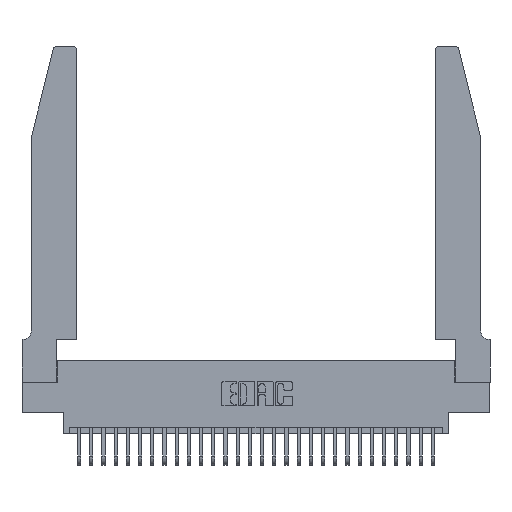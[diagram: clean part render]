
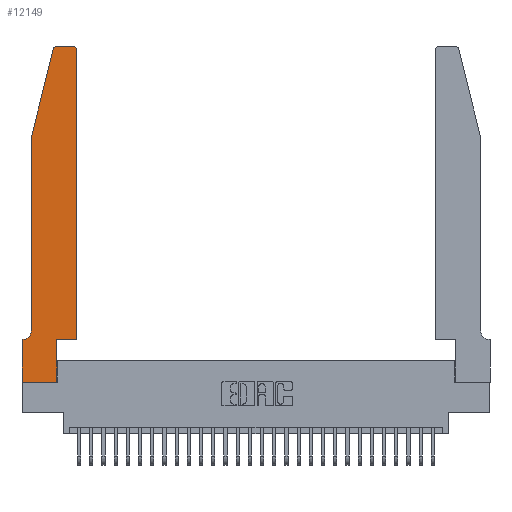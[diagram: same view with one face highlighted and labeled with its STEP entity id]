
A CAD part, top view. The second image highlights one B-rep face of the part: STEP entity #12149.
In plain terms, the highlighted planar face has unit normal (0, 0, 1).
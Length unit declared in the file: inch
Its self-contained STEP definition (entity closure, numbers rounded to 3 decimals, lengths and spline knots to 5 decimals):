
#198 = LINE ( 'NONE', #25534, #5216 ) ;
#710 = DIRECTION ( 'NONE',  ( 0., 0., 1. ) ) ;
#942 = ORIENTED_EDGE ( 'NONE', *, *, #18002, .T. ) ;
#1253 = DIRECTION ( 'NONE',  ( 0., 1., 0. ) ) ;
#2270 = EDGE_CURVE ( 'NONE', #3333, #13601, #4426, .T. ) ;
#2566 = ORIENTED_EDGE ( 'NONE', *, *, #16374, .T. ) ;
#2640 = CARTESIAN_POINT ( 'NONE',  ( 0.0055, 0.42, 0.37 ) ) ;
#3074 = CARTESIAN_POINT ( 'NONE',  ( 0.2865, 0.35, 0.37 ) ) ;
#3125 = DIRECTION ( 'NONE',  ( 0., -1., 0. ) ) ;
#3129 = LINE ( 'NONE', #16320, #8863 ) ;
#3278 = CARTESIAN_POINT ( 'NONE',  ( 0., 0., 0.37 ) ) ;
#3333 = VERTEX_POINT ( 'NONE', #3588 ) ;
#3439 = EDGE_CURVE ( 'NONE', #27283, #3333, #3129, .T. ) ;
#3588 = CARTESIAN_POINT ( 'NONE',  ( 0.0755, 2., 0.37 ) ) ;
#4221 = VECTOR ( 'NONE', #9156, 39.37008 ) ;
#4374 = AXIS2_PLACEMENT_3D ( 'NONE', #2640, #7569, #20020 ) ;
#4426 = LINE ( 'NONE', #17891, #21576 ) ;
#4939 = CARTESIAN_POINT ( 'NONE',  ( 0.4205, 2.75, 0.37 ) ) ;
#4962 = VECTOR ( 'NONE', #5959, 39.37008 ) ;
#5185 = EDGE_CURVE ( 'NONE', #8515, #17104, #23289, .T. ) ;
#5216 = VECTOR ( 'NONE', #20667, 39.37008 ) ;
#5432 = EDGE_CURVE ( 'NONE', #28858, #16392, #21372, .T. ) ;
#5959 = DIRECTION ( 'NONE',  ( -1., 0., 0. ) ) ;
#6767 = CARTESIAN_POINT ( 'NONE',  ( 0., 0.35, 0.37 ) ) ;
#6774 = ORIENTED_EDGE ( 'NONE', *, *, #3439, .T. ) ;
#6834 = CARTESIAN_POINT ( 'NONE',  ( 0.4505, 0.35, 0.37 ) ) ;
#7539 = VECTOR ( 'NONE', #15775, 39.37008 ) ;
#7569 = DIRECTION ( 'NONE',  ( 0., 0., -1. ) ) ;
#7697 = CARTESIAN_POINT ( 'NONE',  ( 0.0755, 0.35, 0.37 ) ) ;
#8092 = CARTESIAN_POINT ( 'NONE',  ( 0., 0., 0.37 ) ) ;
#8168 = ORIENTED_EDGE ( 'NONE', *, *, #5432, .T. ) ;
#8515 = VERTEX_POINT ( 'NONE', #26341 ) ;
#8863 = VECTOR ( 'NONE', #21201, 39.37008 ) ;
#9156 = DIRECTION ( 'NONE',  ( 1., 0., 0. ) ) ;
#9427 = CIRCLE ( 'NONE', #24468, 0.03 ) ;
#10374 = VECTOR ( 'NONE', #20344, 39.37008 ) ;
#11298 = DIRECTION ( 'NONE',  ( 0., 0., 1. ) ) ;
#11558 = EDGE_LOOP ( 'NONE', ( #22653, #24666, #6774, #12377, #27854, #18503, #28241, #942, #14962, #8168, #2566, #25197 ) ) ;
#12023 = EDGE_CURVE ( 'NONE', #13601, #8515, #17518, .T. ) ;
#12140 = VERTEX_POINT ( 'NONE', #4939 ) ;
#12149 = ADVANCED_FACE ( 'NONE', ( #13636 ), #31467, .T. ) ;
#12377 = ORIENTED_EDGE ( 'NONE', *, *, #2270, .T. ) ;
#12439 = EDGE_CURVE ( 'NONE', #31193, #27283, #9427, .T. ) ;
#13601 = VERTEX_POINT ( 'NONE', #31295 ) ;
#13636 = FACE_OUTER_BOUND ( 'NONE', #11558, .T. ) ;
#14403 = DIRECTION ( 'NONE',  ( 1., 0., 0. ) ) ;
#14962 = ORIENTED_EDGE ( 'NONE', *, *, #22237, .T. ) ;
#15775 = DIRECTION ( 'NONE',  ( 0., 1., 0. ) ) ;
#16320 = CARTESIAN_POINT ( 'NONE',  ( 0.0755, 2., 0.37 ) ) ;
#16374 = EDGE_CURVE ( 'NONE', #16392, #16545, #21981, .T. ) ;
#16392 = VERTEX_POINT ( 'NONE', #6834 ) ;
#16545 = VERTEX_POINT ( 'NONE', #17097 ) ;
#16924 = LINE ( 'NONE', #3278, #10374 ) ;
#17097 = CARTESIAN_POINT ( 'NONE',  ( 0.4505, 2.72, 0.37 ) ) ;
#17104 = VERTEX_POINT ( 'NONE', #6767 ) ;
#17518 = CIRCLE ( 'NONE', #4374, 0.07 ) ;
#17891 = CARTESIAN_POINT ( 'NONE',  ( 0.0755, 2., 0.37 ) ) ;
#18002 = EDGE_CURVE ( 'NONE', #24023, #27093, #16924, .T. ) ;
#18503 = ORIENTED_EDGE ( 'NONE', *, *, #5185, .T. ) ;
#19335 = VECTOR ( 'NONE', #25236, 39.37008 ) ;
#19357 = CARTESIAN_POINT ( 'NONE',  ( 0., 0.35, 0.37 ) ) ;
#19857 = CARTESIAN_POINT ( 'NONE',  ( 0., 0., 0.37 ) ) ;
#20020 = DIRECTION ( 'NONE',  ( -1., 0., 0. ) ) ;
#20344 = DIRECTION ( 'NONE',  ( 1., 0., 0. ) ) ;
#20535 = LINE ( 'NONE', #3074, #7539 ) ;
#20667 = DIRECTION ( 'NONE',  ( -1., 0., 0. ) ) ;
#20777 = EDGE_CURVE ( 'NONE', #12140, #31193, #198, .T. ) ;
#21201 = DIRECTION ( 'NONE',  ( -0.239, -0.971, 0. ) ) ;
#21372 = LINE ( 'NONE', #23611, #4221 ) ;
#21449 = DIRECTION ( 'NONE',  ( 1., 0., 0. ) ) ;
#21576 = VECTOR ( 'NONE', #3125, 39.37008 ) ;
#21646 = DIRECTION ( 'NONE',  ( 0., 0., 1. ) ) ;
#21981 = LINE ( 'NONE', #25667, #22342 ) ;
#22177 = AXIS2_PLACEMENT_3D ( 'NONE', #23826, #21646, #14403 ) ;
#22237 = EDGE_CURVE ( 'NONE', #27093, #28858, #20535, .T. ) ;
#22342 = VECTOR ( 'NONE', #1253, 39.37008 ) ;
#22542 = CARTESIAN_POINT ( 'NONE',  ( 0.25487, 2.72718, 0.37 ) ) ;
#22653 = ORIENTED_EDGE ( 'NONE', *, *, #20777, .T. ) ;
#23136 = LINE ( 'NONE', #8092, #19335 ) ;
#23289 = LINE ( 'NONE', #7697, #4962 ) ;
#23611 = CARTESIAN_POINT ( 'NONE',  ( 0.4505, 0.35, 0.37 ) ) ;
#23826 = CARTESIAN_POINT ( 'NONE',  ( 0.4205, 2.72, 0.37 ) ) ;
#24023 = VERTEX_POINT ( 'NONE', #19857 ) ;
#24468 = AXIS2_PLACEMENT_3D ( 'NONE', #28343, #11298, #21449 ) ;
#24479 = CARTESIAN_POINT ( 'NONE',  ( 0.2865, 0., 0.37 ) ) ;
#24666 = ORIENTED_EDGE ( 'NONE', *, *, #12439, .T. ) ;
#25149 = EDGE_CURVE ( 'NONE', #17104, #24023, #23136, .T. ) ;
#25197 = ORIENTED_EDGE ( 'NONE', *, *, #25343, .T. ) ;
#25236 = DIRECTION ( 'NONE',  ( 0., -1., 0. ) ) ;
#25343 = EDGE_CURVE ( 'NONE', #16545, #12140, #26635, .T. ) ;
#25534 = CARTESIAN_POINT ( 'NONE',  ( 0.2605, 2.75, 0.37 ) ) ;
#25667 = CARTESIAN_POINT ( 'NONE',  ( 0.4505, 0.35, 0.37 ) ) ;
#26265 = CARTESIAN_POINT ( 'NONE',  ( 0.284, 2.75, 0.37 ) ) ;
#26341 = CARTESIAN_POINT ( 'NONE',  ( 0.0055, 0.35, 0.37 ) ) ;
#26635 = CIRCLE ( 'NONE', #22177, 0.03 ) ;
#27093 = VERTEX_POINT ( 'NONE', #24479 ) ;
#27283 = VERTEX_POINT ( 'NONE', #22542 ) ;
#27714 = AXIS2_PLACEMENT_3D ( 'NONE', #19357, #710, #30338 ) ;
#27854 = ORIENTED_EDGE ( 'NONE', *, *, #12023, .T. ) ;
#28241 = ORIENTED_EDGE ( 'NONE', *, *, #25149, .T. ) ;
#28343 = CARTESIAN_POINT ( 'NONE',  ( 0.284, 2.72, 0.37 ) ) ;
#28858 = VERTEX_POINT ( 'NONE', #31072 ) ;
#30338 = DIRECTION ( 'NONE',  ( 1., 0., 0. ) ) ;
#31072 = CARTESIAN_POINT ( 'NONE',  ( 0.2865, 0.35, 0.37 ) ) ;
#31193 = VERTEX_POINT ( 'NONE', #26265 ) ;
#31295 = CARTESIAN_POINT ( 'NONE',  ( 0.0755, 0.42, 0.37 ) ) ;
#31467 = PLANE ( 'NONE',  #27714 ) ;
